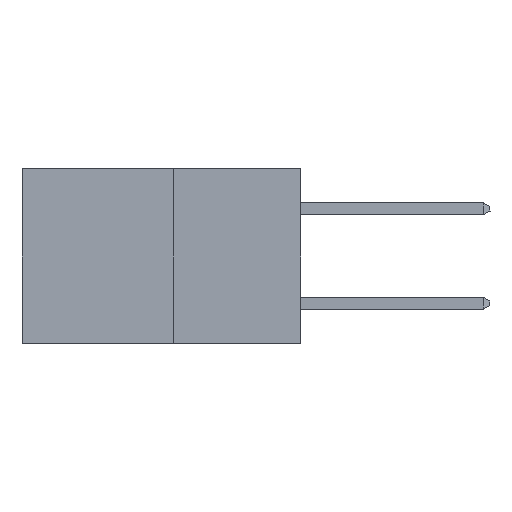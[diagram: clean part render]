
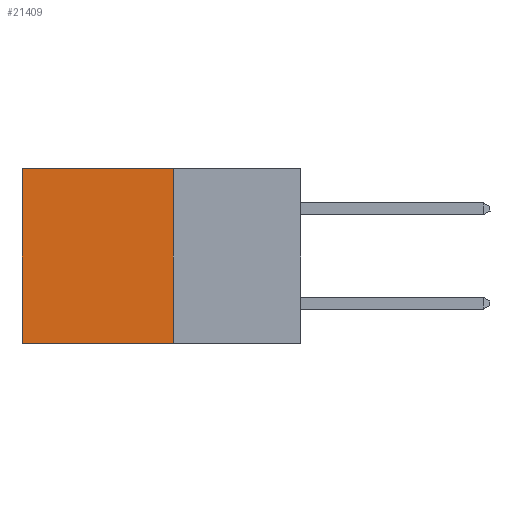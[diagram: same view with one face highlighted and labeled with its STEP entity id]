
A CAD part, left-side view. The second image highlights one B-rep face of the part: STEP entity #21409.
In plain terms, the highlighted planar face has unit normal (-1, 0, 0).
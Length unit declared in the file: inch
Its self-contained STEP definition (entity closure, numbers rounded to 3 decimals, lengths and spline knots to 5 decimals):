
#296 = PLANE ( 'NONE',  #15006 ) ;
#1600 = VERTEX_POINT ( 'NONE', #24457 ) ;
#1942 = DIRECTION ( 'NONE',  ( 0., 0., -1. ) ) ;
#3166 = VERTEX_POINT ( 'NONE', #9726 ) ;
#3863 = CARTESIAN_POINT ( 'NONE',  ( 0.277, 0.59, 0. ) ) ;
#3937 = LINE ( 'NONE', #16002, #25203 ) ;
#4415 = DIRECTION ( 'NONE',  ( 0., 0., -1. ) ) ;
#4643 = EDGE_CURVE ( 'NONE', #1600, #6075, #10832, .T. ) ;
#4833 = ORIENTED_EDGE ( 'NONE', *, *, #7340, .T. ) ;
#4837 = VECTOR ( 'NONE', #19700, 39.37008 ) ;
#5160 = CARTESIAN_POINT ( 'NONE',  ( 0.277, 0.59, -0.37 ) ) ;
#5897 = ORIENTED_EDGE ( 'NONE', *, *, #7139, .T. ) ;
#6075 = VERTEX_POINT ( 'NONE', #5160 ) ;
#7119 = DIRECTION ( 'NONE',  ( 0., 1., 0. ) ) ;
#7139 = EDGE_CURVE ( 'NONE', #3166, #24501, #18995, .T. ) ;
#7340 = EDGE_CURVE ( 'NONE', #24501, #6075, #3937, .T. ) ;
#7573 = CARTESIAN_POINT ( 'NONE',  ( 0.277, 0.27, 0. ) ) ;
#9726 = CARTESIAN_POINT ( 'NONE',  ( 0.277, 0.27, 0. ) ) ;
#10350 = VECTOR ( 'NONE', #17786, 39.37008 ) ;
#10832 = LINE ( 'NONE', #17845, #4837 ) ;
#14399 = CARTESIAN_POINT ( 'NONE',  ( 0.277, 0.27, -0.37 ) ) ;
#14816 = ORIENTED_EDGE ( 'NONE', *, *, #21214, .F. ) ;
#15006 = AXIS2_PLACEMENT_3D ( 'NONE', #14399, #16392, #4415 ) ;
#15059 = EDGE_LOOP ( 'NONE', ( #4833, #18056, #14816, #5897 ) ) ;
#15619 = LINE ( 'NONE', #15712, #10350 ) ;
#15712 = CARTESIAN_POINT ( 'NONE',  ( 0.277, 0.27, -0.37 ) ) ;
#16002 = CARTESIAN_POINT ( 'NONE',  ( 0.277, 0.59, -0.37 ) ) ;
#16392 = DIRECTION ( 'NONE',  ( 1., 0., 0. ) ) ;
#16535 = FACE_OUTER_BOUND ( 'NONE', #15059, .T. ) ;
#17786 = DIRECTION ( 'NONE',  ( 0., 0., -1. ) ) ;
#17845 = CARTESIAN_POINT ( 'NONE',  ( 0.277, 0.27, -0.37 ) ) ;
#18056 = ORIENTED_EDGE ( 'NONE', *, *, #4643, .F. ) ;
#18995 = LINE ( 'NONE', #7573, #19613 ) ;
#19613 = VECTOR ( 'NONE', #7119, 39.37008 ) ;
#19700 = DIRECTION ( 'NONE',  ( 0., 1., 0. ) ) ;
#21214 = EDGE_CURVE ( 'NONE', #3166, #1600, #15619, .T. ) ;
#21409 = ADVANCED_FACE ( 'NONE', ( #16535 ), #296, .F. ) ;
#24457 = CARTESIAN_POINT ( 'NONE',  ( 0.277, 0.27, -0.37 ) ) ;
#24501 = VERTEX_POINT ( 'NONE', #3863 ) ;
#25203 = VECTOR ( 'NONE', #1942, 39.37008 ) ;
